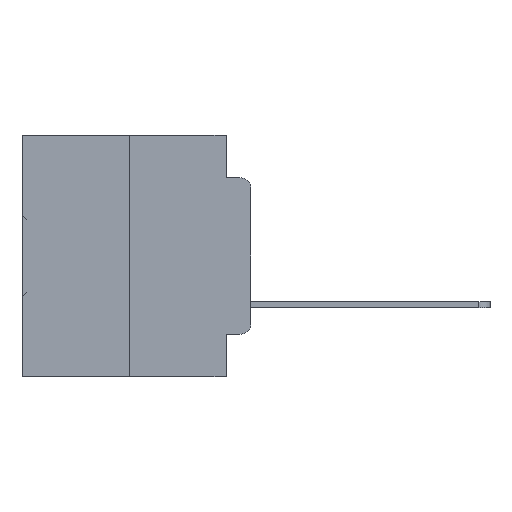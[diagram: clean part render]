
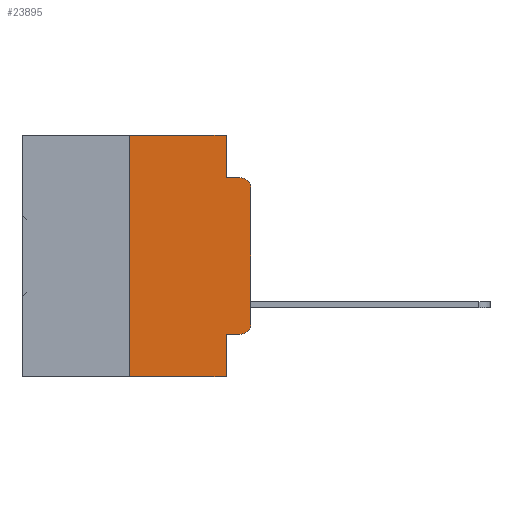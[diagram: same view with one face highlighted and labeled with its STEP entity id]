
A CAD part, left-side view. The second image highlights one B-rep face of the part: STEP entity #23895.
In plain terms, the highlighted planar face has unit normal (-1, 0, 0).
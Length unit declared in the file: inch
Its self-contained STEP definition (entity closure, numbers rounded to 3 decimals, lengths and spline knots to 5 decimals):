
#294 = DIRECTION ( 'NONE',  ( 0., -1., 0. ) ) ;
#303 = ORIENTED_EDGE ( 'NONE', *, *, #14306, .T. ) ;
#762 = ORIENTED_EDGE ( 'NONE', *, *, #9386, .F. ) ;
#926 = EDGE_CURVE ( 'NONE', #33326, #10405, #21588, .T. ) ;
#1023 = DIRECTION ( 'NONE',  ( 0., -1., 0. ) ) ;
#1705 = CARTESIAN_POINT ( 'NONE',  ( 0., 0., 0. ) ) ;
#2884 = VECTOR ( 'NONE', #1023, 39.37008 ) ;
#2894 = DIRECTION ( 'NONE',  ( -1., 0., 0. ) ) ;
#3180 = LINE ( 'NONE', #19994, #26403 ) ;
#4565 = VERTEX_POINT ( 'NONE', #34073 ) ;
#5020 = PLANE ( 'NONE',  #33189 ) ;
#5501 = CIRCLE ( 'NONE', #27188, 0.02 ) ;
#6745 = CARTESIAN_POINT ( 'NONE',  ( 0., 0.25, -0.5 ) ) ;
#8488 = LINE ( 'NONE', #12785, #15703 ) ;
#9386 = EDGE_CURVE ( 'NONE', #10405, #13232, #19513, .T. ) ;
#10405 = VERTEX_POINT ( 'NONE', #13815 ) ;
#10956 = EDGE_CURVE ( 'NONE', #15068, #11822, #11222, .T. ) ;
#11177 = EDGE_CURVE ( 'NONE', #4565, #33326, #25670, .T. ) ;
#11222 = LINE ( 'NONE', #31149, #2884 ) ;
#11316 = LINE ( 'NONE', #1705, #25313 ) ;
#11539 = FACE_OUTER_BOUND ( 'NONE', #32736, .T. ) ;
#11822 = VERTEX_POINT ( 'NONE', #36805 ) ;
#12785 = CARTESIAN_POINT ( 'NONE',  ( 0., 0.051, -0.4115 ) ) ;
#12909 = CARTESIAN_POINT ( 'NONE',  ( 0., 0.02, -0.4115 ) ) ;
#13128 = CARTESIAN_POINT ( 'NONE',  ( 0., 0.02, -0.1085 ) ) ;
#13232 = VERTEX_POINT ( 'NONE', #33614 ) ;
#13650 = VECTOR ( 'NONE', #16368, 39.37008 ) ;
#13815 = CARTESIAN_POINT ( 'NONE',  ( 0., 0.051, -0.0885 ) ) ;
#14296 = DIRECTION ( 'NONE',  ( 0., 0., -1. ) ) ;
#14306 = EDGE_CURVE ( 'NONE', #28373, #24780, #36062, .T. ) ;
#14979 = ORIENTED_EDGE ( 'NONE', *, *, #926, .F. ) ;
#15068 = VERTEX_POINT ( 'NONE', #6745 ) ;
#15608 = EDGE_CURVE ( 'NONE', #27438, #13232, #5501, .T. ) ;
#15703 = VECTOR ( 'NONE', #294, 39.37008 ) ;
#16071 = LINE ( 'NONE', #36067, #23926 ) ;
#16253 = DIRECTION ( 'NONE',  ( 0., 0., -1. ) ) ;
#16368 = DIRECTION ( 'NONE',  ( 0., 0., -1. ) ) ;
#16632 = DIRECTION ( 'NONE',  ( 0., -1., 0. ) ) ;
#16791 = CARTESIAN_POINT ( 'NONE',  ( 0., 0.051, 0. ) ) ;
#16863 = ORIENTED_EDGE ( 'NONE', *, *, #37536, .F. ) ;
#16948 = VECTOR ( 'NONE', #29532, 39.37008 ) ;
#17648 = EDGE_CURVE ( 'NONE', #24780, #27438, #11316, .T. ) ;
#18580 = VECTOR ( 'NONE', #16632, 39.37008 ) ;
#18701 = ORIENTED_EDGE ( 'NONE', *, *, #10956, .T. ) ;
#18864 = DIRECTION ( 'NONE',  ( 0., 0., -1. ) ) ;
#18973 = VERTEX_POINT ( 'NONE', #36064 ) ;
#19513 = LINE ( 'NONE', #28167, #18580 ) ;
#19994 = CARTESIAN_POINT ( 'NONE',  ( 0., 0.25, 0. ) ) ;
#21233 = CARTESIAN_POINT ( 'NONE',  ( 0., 0.02, -0.3915 ) ) ;
#21588 = LINE ( 'NONE', #33791, #13650 ) ;
#22402 = ORIENTED_EDGE ( 'NONE', *, *, #15608, .T. ) ;
#23895 = ADVANCED_FACE ( 'NONE', ( #11539 ), #5020, .F. ) ;
#23926 = VECTOR ( 'NONE', #18864, 39.37008 ) ;
#24197 = DIRECTION ( 'NONE',  ( 0., 0., -1. ) ) ;
#24780 = VERTEX_POINT ( 'NONE', #35597 ) ;
#25313 = VECTOR ( 'NONE', #34574, 39.37008 ) ;
#25670 = LINE ( 'NONE', #29414, #16948 ) ;
#26403 = VECTOR ( 'NONE', #28810, 39.37008 ) ;
#27188 = AXIS2_PLACEMENT_3D ( 'NONE', #13128, #33691, #16253 ) ;
#27438 = VERTEX_POINT ( 'NONE', #35376 ) ;
#28167 = CARTESIAN_POINT ( 'NONE',  ( 0., 0.051, -0.0885 ) ) ;
#28373 = VERTEX_POINT ( 'NONE', #12909 ) ;
#28379 = ORIENTED_EDGE ( 'NONE', *, *, #11177, .F. ) ;
#28810 = DIRECTION ( 'NONE',  ( 0., 0., 1. ) ) ;
#28845 = ORIENTED_EDGE ( 'NONE', *, *, #30116, .T. ) ;
#29036 = CARTESIAN_POINT ( 'NONE',  ( 0., 0.473, 0. ) ) ;
#29414 = CARTESIAN_POINT ( 'NONE',  ( 0., 0.473, 0. ) ) ;
#29532 = DIRECTION ( 'NONE',  ( 0., -1., 0. ) ) ;
#30116 = EDGE_CURVE ( 'NONE', #18973, #28373, #8488, .T. ) ;
#31149 = CARTESIAN_POINT ( 'NONE',  ( 0., 0.473, -0.5 ) ) ;
#31931 = DIRECTION ( 'NONE',  ( 1., 0., 0. ) ) ;
#32736 = EDGE_LOOP ( 'NONE', ( #37055, #22402, #762, #14979, #28379, #16863, #18701, #35448, #28845, #303 ) ) ;
#33189 = AXIS2_PLACEMENT_3D ( 'NONE', #29036, #31931, #14296 ) ;
#33326 = VERTEX_POINT ( 'NONE', #16791 ) ;
#33614 = CARTESIAN_POINT ( 'NONE',  ( 0., 0.02, -0.0885 ) ) ;
#33691 = DIRECTION ( 'NONE',  ( -1., 0., 0. ) ) ;
#33791 = CARTESIAN_POINT ( 'NONE',  ( 0., 0.051, 0. ) ) ;
#33935 = EDGE_CURVE ( 'NONE', #18973, #11822, #16071, .T. ) ;
#34073 = CARTESIAN_POINT ( 'NONE',  ( 0., 0.25, 0. ) ) ;
#34574 = DIRECTION ( 'NONE',  ( 0., 0., 1. ) ) ;
#35376 = CARTESIAN_POINT ( 'NONE',  ( 0., 0., -0.1085 ) ) ;
#35448 = ORIENTED_EDGE ( 'NONE', *, *, #33935, .F. ) ;
#35597 = CARTESIAN_POINT ( 'NONE',  ( 0., 0., -0.3915 ) ) ;
#36062 = CIRCLE ( 'NONE', #38352, 0.02 ) ;
#36064 = CARTESIAN_POINT ( 'NONE',  ( 0., 0.051, -0.4115 ) ) ;
#36067 = CARTESIAN_POINT ( 'NONE',  ( 0., 0.051, 0. ) ) ;
#36805 = CARTESIAN_POINT ( 'NONE',  ( 0., 0.051, -0.5 ) ) ;
#37055 = ORIENTED_EDGE ( 'NONE', *, *, #17648, .T. ) ;
#37536 = EDGE_CURVE ( 'NONE', #15068, #4565, #3180, .T. ) ;
#38352 = AXIS2_PLACEMENT_3D ( 'NONE', #21233, #2894, #24197 ) ;
